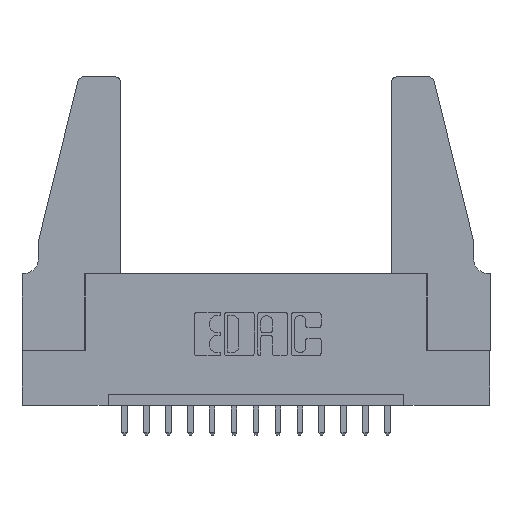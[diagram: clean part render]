
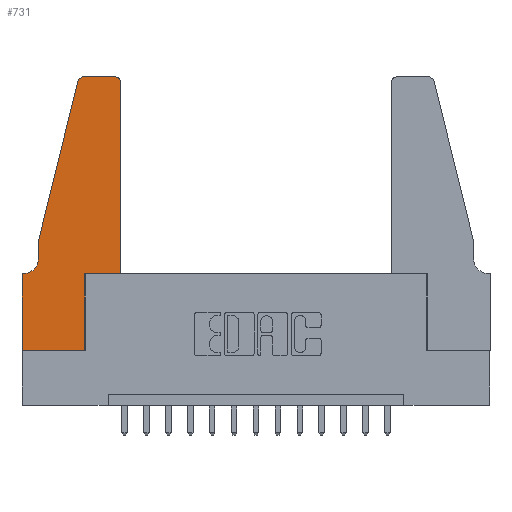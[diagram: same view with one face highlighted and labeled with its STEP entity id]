
A CAD part, top view. The second image highlights one B-rep face of the part: STEP entity #731.
In plain terms, the highlighted planar face has unit normal (0, 0, 1).
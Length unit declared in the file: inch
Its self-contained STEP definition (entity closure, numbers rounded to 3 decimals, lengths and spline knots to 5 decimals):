
#235 = EDGE_CURVE ( 'NONE', #9250, #5323, #1767, .T. ) ;
#247 = VECTOR ( 'NONE', #1979, 39.37008 ) ;
#455 = VERTEX_POINT ( 'NONE', #9100 ) ;
#541 = CIRCLE ( 'NONE', #13939, 0.07 ) ;
#611 = CARTESIAN_POINT ( 'NONE',  ( 0.4205, 1.22, 0.37 ) ) ;
#731 = ADVANCED_FACE ( 'NONE', ( #5770 ), #13580, .T. ) ;
#775 = CARTESIAN_POINT ( 'NONE',  ( 0.0755, 0.5, 0.37 ) ) ;
#937 = CARTESIAN_POINT ( 'NONE',  ( 0.0755, 0.35, 0.37 ) ) ;
#954 = CIRCLE ( 'NONE', #8203, 0.03 ) ;
#1113 = ORIENTED_EDGE ( 'NONE', *, *, #5322, .T. ) ;
#1257 = ORIENTED_EDGE ( 'NONE', *, *, #10279, .T. ) ;
#1331 = EDGE_CURVE ( 'NONE', #12904, #13045, #3846, .T. ) ;
#1501 = DIRECTION ( 'NONE',  ( 1., 0., 0. ) ) ;
#1626 = DIRECTION ( 'NONE',  ( 1., 0., 0. ) ) ;
#1767 = LINE ( 'NONE', #11724, #247 ) ;
#1979 = DIRECTION ( 'NONE',  ( -0.239, -0.971, 0. ) ) ;
#1984 = LINE ( 'NONE', #775, #3323 ) ;
#2191 = VECTOR ( 'NONE', #5790, 39.37008 ) ;
#2284 = CARTESIAN_POINT ( 'NONE',  ( 0.4205, 1.25, 0.37 ) ) ;
#2292 = DIRECTION ( 'NONE',  ( 0., -1., 0. ) ) ;
#2880 = LINE ( 'NONE', #9687, #8611 ) ;
#2909 = ORIENTED_EDGE ( 'NONE', *, *, #4924, .T. ) ;
#3261 = CARTESIAN_POINT ( 'NONE',  ( 0.0055, 0.42, 0.37 ) ) ;
#3323 = VECTOR ( 'NONE', #14118, 39.37008 ) ;
#3537 = LINE ( 'NONE', #937, #2191 ) ;
#3846 = LINE ( 'NONE', #10894, #7477 ) ;
#3848 = CARTESIAN_POINT ( 'NONE',  ( 0.0755, 0.5, 0.37 ) ) ;
#3879 = ORIENTED_EDGE ( 'NONE', *, *, #14247, .T. ) ;
#4040 = ORIENTED_EDGE ( 'NONE', *, *, #8984, .T. ) ;
#4811 = DIRECTION ( 'NONE',  ( 0., 0., 1. ) ) ;
#4924 = EDGE_CURVE ( 'NONE', #455, #12532, #6524, .T. ) ;
#5219 = ORIENTED_EDGE ( 'NONE', *, *, #15364, .T. ) ;
#5322 = EDGE_CURVE ( 'NONE', #12532, #12904, #10905, .T. ) ;
#5323 = VERTEX_POINT ( 'NONE', #3848 ) ;
#5591 = AXIS2_PLACEMENT_3D ( 'NONE', #8453, #4811, #8347 ) ;
#5770 = FACE_OUTER_BOUND ( 'NONE', #7265, .T. ) ;
#5790 = DIRECTION ( 'NONE',  ( -1., 0., 0. ) ) ;
#5900 = VECTOR ( 'NONE', #2292, 39.37008 ) ;
#5937 = CARTESIAN_POINT ( 'NONE',  ( 0.0055, 0.35, 0.37 ) ) ;
#6023 = CARTESIAN_POINT ( 'NONE',  ( 0., 0.35, 0.37 ) ) ;
#6524 = LINE ( 'NONE', #14845, #11288 ) ;
#7265 = EDGE_LOOP ( 'NONE', ( #13687, #1257, #11164, #11062, #12874, #9817, #4040, #5219, #2909, #1113, #14400, #3879 ) ) ;
#7477 = VECTOR ( 'NONE', #14599, 39.37008 ) ;
#7755 = EDGE_CURVE ( 'NONE', #11376, #12024, #3537, .T. ) ;
#7926 = DIRECTION ( 'NONE',  ( 0., 0., 1. ) ) ;
#8203 = AXIS2_PLACEMENT_3D ( 'NONE', #611, #7926, #1626 ) ;
#8347 = DIRECTION ( 'NONE',  ( 1., 0., 0. ) ) ;
#8363 = VECTOR ( 'NONE', #14791, 39.37008 ) ;
#8453 = CARTESIAN_POINT ( 'NONE',  ( 0.284, 1.22, 0.37 ) ) ;
#8531 = CARTESIAN_POINT ( 'NONE',  ( 0., 0., 0.37 ) ) ;
#8611 = VECTOR ( 'NONE', #11296, 39.37008 ) ;
#8868 = CARTESIAN_POINT ( 'NONE',  ( 0.4505, 0.35, 0.37 ) ) ;
#8984 = EDGE_CURVE ( 'NONE', #12024, #12365, #9335, .T. ) ;
#9100 = CARTESIAN_POINT ( 'NONE',  ( 0.2865, 0., 0.37 ) ) ;
#9102 = EDGE_CURVE ( 'NONE', #14341, #11376, #541, .T. ) ;
#9154 = CARTESIAN_POINT ( 'NONE',  ( 0.2865, 0.35, 0.37 ) ) ;
#9250 = VERTEX_POINT ( 'NONE', #13870 ) ;
#9335 = LINE ( 'NONE', #9616, #5900 ) ;
#9364 = CARTESIAN_POINT ( 'NONE',  ( 0.0755, 0.42, 0.37 ) ) ;
#9448 = DIRECTION ( 'NONE',  ( 0., 0., -1. ) ) ;
#9616 = CARTESIAN_POINT ( 'NONE',  ( 0., 0., 0.37 ) ) ;
#9687 = CARTESIAN_POINT ( 'NONE',  ( 0.2605, 1.25, 0.37 ) ) ;
#9742 = CARTESIAN_POINT ( 'NONE',  ( 0., 0.35, 0.37 ) ) ;
#9817 = ORIENTED_EDGE ( 'NONE', *, *, #7755, .T. ) ;
#9886 = CARTESIAN_POINT ( 'NONE',  ( 0.4505, 0.35, 0.37 ) ) ;
#10279 = EDGE_CURVE ( 'NONE', #13015, #9250, #11599, .T. ) ;
#10479 = DIRECTION ( 'NONE',  ( -1., 0., 0. ) ) ;
#10894 = CARTESIAN_POINT ( 'NONE',  ( 0.4505, 0.35, 0.37 ) ) ;
#10905 = LINE ( 'NONE', #8868, #14000 ) ;
#11062 = ORIENTED_EDGE ( 'NONE', *, *, #11295, .T. ) ;
#11096 = DIRECTION ( 'NONE',  ( 1., 0., 0. ) ) ;
#11164 = ORIENTED_EDGE ( 'NONE', *, *, #235, .T. ) ;
#11273 = VERTEX_POINT ( 'NONE', #2284 ) ;
#11288 = VECTOR ( 'NONE', #12726, 39.37008 ) ;
#11295 = EDGE_CURVE ( 'NONE', #5323, #14341, #1984, .T. ) ;
#11296 = DIRECTION ( 'NONE',  ( -1., 0., 0. ) ) ;
#11376 = VERTEX_POINT ( 'NONE', #5937 ) ;
#11393 = CARTESIAN_POINT ( 'NONE',  ( 0.284, 1.25, 0.37 ) ) ;
#11434 = LINE ( 'NONE', #8531, #8363 ) ;
#11599 = CIRCLE ( 'NONE', #5591, 0.03 ) ;
#11724 = CARTESIAN_POINT ( 'NONE',  ( 0.0755, 0.5, 0.37 ) ) ;
#12024 = VERTEX_POINT ( 'NONE', #6023 ) ;
#12365 = VERTEX_POINT ( 'NONE', #12502 ) ;
#12502 = CARTESIAN_POINT ( 'NONE',  ( 0., 0., 0.37 ) ) ;
#12532 = VERTEX_POINT ( 'NONE', #9154 ) ;
#12648 = CARTESIAN_POINT ( 'NONE',  ( 0.4505, 1.22, 0.37 ) ) ;
#12726 = DIRECTION ( 'NONE',  ( 0., 1., 0. ) ) ;
#12874 = ORIENTED_EDGE ( 'NONE', *, *, #9102, .T. ) ;
#12904 = VERTEX_POINT ( 'NONE', #9886 ) ;
#13015 = VERTEX_POINT ( 'NONE', #11393 ) ;
#13045 = VERTEX_POINT ( 'NONE', #12648 ) ;
#13580 = PLANE ( 'NONE',  #14244 ) ;
#13687 = ORIENTED_EDGE ( 'NONE', *, *, #14191, .T. ) ;
#13870 = CARTESIAN_POINT ( 'NONE',  ( 0.25487, 1.22718, 0.37 ) ) ;
#13939 = AXIS2_PLACEMENT_3D ( 'NONE', #3261, #9448, #10479 ) ;
#14000 = VECTOR ( 'NONE', #1501, 39.37008 ) ;
#14118 = DIRECTION ( 'NONE',  ( 0., -1., 0. ) ) ;
#14191 = EDGE_CURVE ( 'NONE', #11273, #13015, #2880, .T. ) ;
#14244 = AXIS2_PLACEMENT_3D ( 'NONE', #9742, #14642, #11096 ) ;
#14247 = EDGE_CURVE ( 'NONE', #13045, #11273, #954, .T. ) ;
#14341 = VERTEX_POINT ( 'NONE', #9364 ) ;
#14400 = ORIENTED_EDGE ( 'NONE', *, *, #1331, .T. ) ;
#14599 = DIRECTION ( 'NONE',  ( 0., 1., 0. ) ) ;
#14642 = DIRECTION ( 'NONE',  ( 0., 0., 1. ) ) ;
#14791 = DIRECTION ( 'NONE',  ( 1., 0., 0. ) ) ;
#14845 = CARTESIAN_POINT ( 'NONE',  ( 0.2865, 0.35, 0.37 ) ) ;
#15364 = EDGE_CURVE ( 'NONE', #12365, #455, #11434, .T. ) ;
